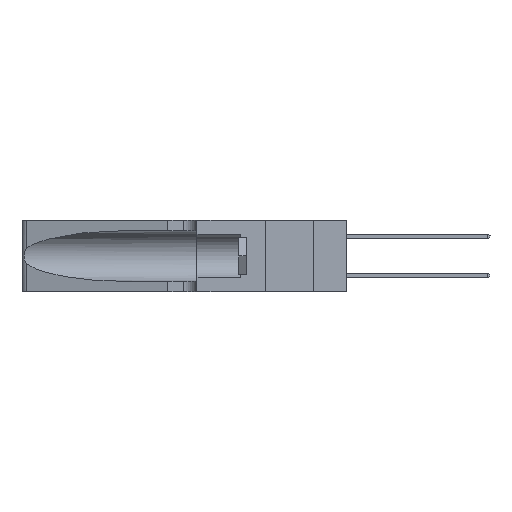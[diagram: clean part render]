
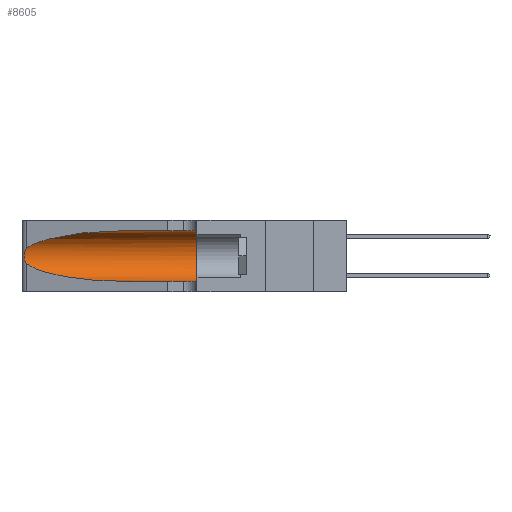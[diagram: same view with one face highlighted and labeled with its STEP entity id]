
A CAD part, left-side view. The second image highlights one B-rep face of the part: STEP entity #8605.
In plain terms, the highlighted cylindrical face has radius 3.308 mm (diameter 6.617 mm), a partial arc.
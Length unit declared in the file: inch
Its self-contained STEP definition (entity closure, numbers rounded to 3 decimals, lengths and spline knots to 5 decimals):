
#893 = DIRECTION ( 'NONE',  ( 0., 1., 0. ) ) ;
#1290 = CARTESIAN_POINT ( 'NONE',  ( 0.25639, 1.23184, 0.21858 ) ) ;
#2287 = LINE ( 'NONE', #39850, #39775 ) ;
#3145 = ORIENTED_EDGE ( 'NONE', *, *, #34747, .T. ) ;
#3521 = CARTESIAN_POINT ( 'NONE',  ( 0.25487, 1.22718, 0.22369 ) ) ;
#4970 = CARTESIAN_POINT ( 'NONE',  ( 0.25854, 1.2359, 0.20912 ) ) ;
#4972 = EDGE_LOOP ( 'NONE', ( #3145, #30735, #9128, #11633, #9394, #29961 ) ) ;
#4995 = DIRECTION ( 'NONE',  ( 0., 0., -1. ) ) ;
#5792 = EDGE_CURVE ( 'NONE', #34578, #28425, #26639, .T. ) ;
#6236 = AXIS2_PLACEMENT_3D ( 'NONE', #22778, #893, #26401 ) ;
#6372 = CARTESIAN_POINT ( 'NONE',  ( 0.2373, 1.15595, 0.28018 ) ) ;
#8283 = EDGE_CURVE ( 'NONE', #42455, #9810, #18425, .T. ) ;
#8605 = ADVANCED_FACE ( 'NONE', ( #39406 ), #10534, .F. ) ;
#8686 = CARTESIAN_POINT ( 'NONE',  ( 0.26075, 1.23896, 0.19203 ) ) ;
#8711 = DIRECTION ( 'NONE',  ( 0., -1., 0. ) ) ;
#9128 = ORIENTED_EDGE ( 'NONE', *, *, #8283, .T. ) ;
#9394 = ORIENTED_EDGE ( 'NONE', *, *, #44718, .F. ) ;
#9444 = CARTESIAN_POINT ( 'NONE',  ( 0.1305, 0.35, 0.31525 ) ) ;
#9810 = VERTEX_POINT ( 'NONE', #40425 ) ;
#9852 = VERTEX_POINT ( 'NONE', #11820 ) ;
#9883 = AXIS2_PLACEMENT_3D ( 'NONE', #30450, #8711, #4995 ) ;
#9927 = B_SPLINE_CURVE_WITH_KNOTS ( 'NONE', 3,
 ( #15869, #12221, #1290, #26784, #4970, #30430, #8686, #34062, #12375, #37688, #16026, #41282, #19670, #44897 ),
 .UNSPECIFIED., .F., .F.,
 ( 4, 2, 2, 2, 2, 2, 4 ),
 ( 0., 0.00027, 0.00053, 0.00107, 0.0016, 0.00187, 0.00214 ),
 .UNSPECIFIED. ) ;
#10534 = CYLINDRICAL_SURFACE ( 'NONE', #9883, 0.13025 ) ;
#11633 = ORIENTED_EDGE ( 'NONE', *, *, #29764, .T. ) ;
#11820 = CARTESIAN_POINT ( 'NONE',  ( 0.1305, 0.35, 0.05475 ) ) ;
#12221 = CARTESIAN_POINT ( 'NONE',  ( 0.25555, 1.22994, 0.2215 ) ) ;
#12375 = CARTESIAN_POINT ( 'NONE',  ( 0.26017, 1.23833, 0.17102 ) ) ;
#15869 = CARTESIAN_POINT ( 'NONE',  ( 0.25487, 1.22718, 0.22369 ) ) ;
#15876 = VECTOR ( 'NONE', #31143, 39.37008 ) ;
#16026 = CARTESIAN_POINT ( 'NONE',  ( 0.25789, 1.23486, 0.15765 ) ) ;
#16451 = CARTESIAN_POINT ( 'NONE',  ( 0.1305, 0.72297, 0.31525 ) ) ;
#17243 = CARTESIAN_POINT ( 'NONE',  ( 0.18966, 0.96281, 0.31525 ) ) ;
#18425 =( BOUNDED_CURVE ( )  B_SPLINE_CURVE ( 3, ( #21657, #43239, #46854, #25251 ),
 .UNSPECIFIED., .F., .F. ) 
 B_SPLINE_CURVE_WITH_KNOTS ( ( 4, 4 ),
 ( 3.44316, 4.71239 ),
 .UNSPECIFIED. ) 
 CURVE ( )  GEOMETRIC_REPRESENTATION_ITEM ( )  RATIONAL_B_SPLINE_CURVE ( ( 1., 0.87, 0.87, 1. ) ) 
 REPRESENTATION_ITEM ( '' )  );
#19385 = EDGE_CURVE ( 'NONE', #37757, #42455, #9927, .T. ) ;
#19670 = CARTESIAN_POINT ( 'NONE',  ( 0.25555, 1.22993, 0.14849 ) ) ;
#21657 = CARTESIAN_POINT ( 'NONE',  ( 0.25487, 1.22718, 0.14631 ) ) ;
#22778 = CARTESIAN_POINT ( 'NONE',  ( 0.1305, 0.35, 0.185 ) ) ;
#25251 = CARTESIAN_POINT ( 'NONE',  ( 0.1305, 0.72297, 0.05475 ) ) ;
#26401 = DIRECTION ( 'NONE',  ( 0., 0., 1. ) ) ;
#26639 = LINE ( 'NONE', #34638, #15876 ) ;
#26784 = CARTESIAN_POINT ( 'NONE',  ( 0.25787, 1.23484, 0.2124 ) ) ;
#28425 = VERTEX_POINT ( 'NONE', #9444 ) ;
#29764 = EDGE_CURVE ( 'NONE', #9810, #9852, #2287, .T. ) ;
#29961 = ORIENTED_EDGE ( 'NONE', *, *, #5792, .F. ) ;
#30430 = CARTESIAN_POINT ( 'NONE',  ( 0.26018, 1.23835, 0.19895 ) ) ;
#30450 = CARTESIAN_POINT ( 'NONE',  ( 0.1305, 1.61858, 0.185 ) ) ;
#30735 = ORIENTED_EDGE ( 'NONE', *, *, #19385, .T. ) ;
#31143 = DIRECTION ( 'NONE',  ( 0., -1., 0. ) ) ;
#31772 = CARTESIAN_POINT ( 'NONE',  ( 0.25487, 1.22718, 0.22369 ) ) ;
#34062 = CARTESIAN_POINT ( 'NONE',  ( 0.26075, 1.23896, 0.178 ) ) ;
#34578 = VERTEX_POINT ( 'NONE', #16451 ) ;
#34638 = CARTESIAN_POINT ( 'NONE',  ( 0.1305, 1.61858, 0.31525 ) ) ;
#34747 = EDGE_CURVE ( 'NONE', #34578, #37757, #45001, .T. ) ;
#37688 = CARTESIAN_POINT ( 'NONE',  ( 0.25856, 1.23593, 0.16098 ) ) ;
#37757 = VERTEX_POINT ( 'NONE', #3521 ) ;
#38231 = CARTESIAN_POINT ( 'NONE',  ( 0.25487, 1.22718, 0.14631 ) ) ;
#39406 = FACE_OUTER_BOUND ( 'NONE', #4972, .T. ) ;
#39775 = VECTOR ( 'NONE', #43479, 39.37008 ) ;
#39850 = CARTESIAN_POINT ( 'NONE',  ( 0.1305, 1.61858, 0.05475 ) ) ;
#40425 = CARTESIAN_POINT ( 'NONE',  ( 0.1305, 0.72297, 0.05475 ) ) ;
#41282 = CARTESIAN_POINT ( 'NONE',  ( 0.25639, 1.23186, 0.15144 ) ) ;
#42455 = VERTEX_POINT ( 'NONE', #38231 ) ;
#42496 = CARTESIAN_POINT ( 'NONE',  ( 0.1305, 0.72297, 0.31525 ) ) ;
#43239 = CARTESIAN_POINT ( 'NONE',  ( 0.2373, 1.15595, 0.08982 ) ) ;
#43479 = DIRECTION ( 'NONE',  ( 0., -1., 0. ) ) ;
#44718 = EDGE_CURVE ( 'NONE', #28425, #9852, #46639, .T. ) ;
#44897 = CARTESIAN_POINT ( 'NONE',  ( 0.25487, 1.22718, 0.14631 ) ) ;
#45001 =( BOUNDED_CURVE ( )  B_SPLINE_CURVE ( 3, ( #42496, #17243, #6372, #31772 ),
 .UNSPECIFIED., .F., .F. ) 
 B_SPLINE_CURVE_WITH_KNOTS ( ( 4, 4 ),
 ( 1.5708, 2.84003 ),
 .UNSPECIFIED. ) 
 CURVE ( )  GEOMETRIC_REPRESENTATION_ITEM ( )  RATIONAL_B_SPLINE_CURVE ( ( 1., 0.87, 0.87, 1. ) ) 
 REPRESENTATION_ITEM ( '' )  );
#46639 = CIRCLE ( 'NONE', #6236, 0.13025 ) ;
#46854 = CARTESIAN_POINT ( 'NONE',  ( 0.18966, 0.96281, 0.05475 ) ) ;
